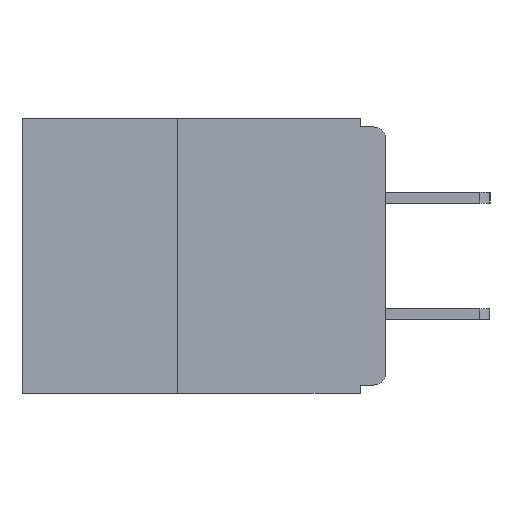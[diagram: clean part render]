
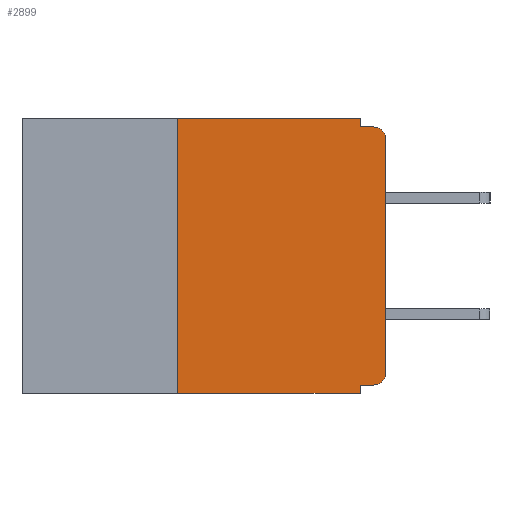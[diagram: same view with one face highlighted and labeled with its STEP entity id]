
A CAD part, left-side view. The second image highlights one B-rep face of the part: STEP entity #2899.
In plain terms, the highlighted planar face has unit normal (-1, 0, 0).
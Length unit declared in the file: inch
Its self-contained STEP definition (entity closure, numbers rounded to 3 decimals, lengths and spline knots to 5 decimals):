
#311 = VECTOR ( 'NONE', #7540, 39.37008 ) ;
#428 = CARTESIAN_POINT ( 'NONE',  ( 0., 0.25, 0. ) ) ;
#472 = VECTOR ( 'NONE', #2282, 39.37008 ) ;
#618 = CARTESIAN_POINT ( 'NONE',  ( 0., 0.015, -0.32 ) ) ;
#641 = VECTOR ( 'NONE', #3483, 39.37008 ) ;
#679 = EDGE_CURVE ( 'NONE', #4457, #3249, #1310, .T. ) ;
#715 = CARTESIAN_POINT ( 'NONE',  ( 0., 0., -0.32 ) ) ;
#743 = ORIENTED_EDGE ( 'NONE', *, *, #795, .T. ) ;
#750 = EDGE_CURVE ( 'NONE', #2171, #4228, #9390, .T. ) ;
#795 = EDGE_CURVE ( 'NONE', #2171, #6616, #3520, .T. ) ;
#797 = LINE ( 'NONE', #11637, #472 ) ;
#818 = EDGE_CURVE ( 'NONE', #1198, #6616, #797, .T. ) ;
#1198 = VERTEX_POINT ( 'NONE', #11765 ) ;
#1310 = LINE ( 'NONE', #1751, #311 ) ;
#1383 = VECTOR ( 'NONE', #2618, 39.37008 ) ;
#1410 = ORIENTED_EDGE ( 'NONE', *, *, #6175, .T. ) ;
#1751 = CARTESIAN_POINT ( 'NONE',  ( 0., 0.031, 0. ) ) ;
#1775 = AXIS2_PLACEMENT_3D ( 'NONE', #5430, #5412, #5399 ) ;
#1803 = VECTOR ( 'NONE', #10834, 39.37008 ) ;
#1867 = LINE ( 'NONE', #715, #9729 ) ;
#2171 = VERTEX_POINT ( 'NONE', #10410 ) ;
#2282 = DIRECTION ( 'NONE',  ( 0., 0., -1. ) ) ;
#2454 = DIRECTION ( 'NONE',  ( -1., 0., 0. ) ) ;
#2488 = CARTESIAN_POINT ( 'NONE',  ( 0., 0.437, 0. ) ) ;
#2618 = DIRECTION ( 'NONE',  ( 0., -1., 0. ) ) ;
#2655 = CARTESIAN_POINT ( 'NONE',  ( 0., 0.031, -0.01 ) ) ;
#2899 = ADVANCED_FACE ( 'NONE', ( #3017 ), #5442, .F. ) ;
#2933 = CARTESIAN_POINT ( 'NONE',  ( 0., 0.25, -0.33 ) ) ;
#3017 = FACE_OUTER_BOUND ( 'NONE', #11963, .T. ) ;
#3060 = VECTOR ( 'NONE', #6805, 39.37008 ) ;
#3136 = VERTEX_POINT ( 'NONE', #3401 ) ;
#3249 = VERTEX_POINT ( 'NONE', #2655 ) ;
#3401 = CARTESIAN_POINT ( 'NONE',  ( 0., 0., -0.305 ) ) ;
#3478 = ORIENTED_EDGE ( 'NONE', *, *, #818, .F. ) ;
#3483 = DIRECTION ( 'NONE',  ( 0., -1., 0. ) ) ;
#3520 = LINE ( 'NONE', #11649, #6071 ) ;
#3541 = CARTESIAN_POINT ( 'NONE',  ( 0., 0.031, -0.33 ) ) ;
#4062 = ORIENTED_EDGE ( 'NONE', *, *, #9400, .T. ) ;
#4228 = VERTEX_POINT ( 'NONE', #428 ) ;
#4290 = CARTESIAN_POINT ( 'NONE',  ( 0., 0.015, -0.305 ) ) ;
#4457 = VERTEX_POINT ( 'NONE', #10857 ) ;
#5075 = AXIS2_PLACEMENT_3D ( 'NONE', #4290, #10738, #5265 ) ;
#5265 = DIRECTION ( 'NONE',  ( 0., 0., -1. ) ) ;
#5294 = ORIENTED_EDGE ( 'NONE', *, *, #10520, .T. ) ;
#5322 = CARTESIAN_POINT ( 'NONE',  ( 0., 0.015, -0.01 ) ) ;
#5399 = DIRECTION ( 'NONE',  ( 0., 0., -1. ) ) ;
#5412 = DIRECTION ( 'NONE',  ( 1., 0., 0. ) ) ;
#5430 = CARTESIAN_POINT ( 'NONE',  ( 0., 0.437, 0. ) ) ;
#5441 = ORIENTED_EDGE ( 'NONE', *, *, #750, .F. ) ;
#5442 = PLANE ( 'NONE',  #1775 ) ;
#5630 = LINE ( 'NONE', #8663, #3060 ) ;
#6071 = VECTOR ( 'NONE', #9850, 39.37008 ) ;
#6175 = EDGE_CURVE ( 'NONE', #3136, #7165, #5630, .T. ) ;
#6616 = VERTEX_POINT ( 'NONE', #3541 ) ;
#6631 = DIRECTION ( 'NONE',  ( 0., 1., 0. ) ) ;
#6805 = DIRECTION ( 'NONE',  ( 0., 0., 1. ) ) ;
#6875 = LINE ( 'NONE', #10138, #1383 ) ;
#7045 = ORIENTED_EDGE ( 'NONE', *, *, #10639, .F. ) ;
#7165 = VERTEX_POINT ( 'NONE', #9878 ) ;
#7174 = ORIENTED_EDGE ( 'NONE', *, *, #679, .F. ) ;
#7386 = EDGE_CURVE ( 'NONE', #3249, #8506, #6875, .T. ) ;
#7540 = DIRECTION ( 'NONE',  ( 0., 0., -1. ) ) ;
#7552 = CIRCLE ( 'NONE', #10906, 0.015 ) ;
#8198 = CARTESIAN_POINT ( 'NONE',  ( 0., 0.015, -0.025 ) ) ;
#8506 = VERTEX_POINT ( 'NONE', #5322 ) ;
#8663 = CARTESIAN_POINT ( 'NONE',  ( 0., 0., 0. ) ) ;
#8858 = EDGE_CURVE ( 'NONE', #11752, #1198, #1867, .T. ) ;
#9009 = LINE ( 'NONE', #2488, #641 ) ;
#9090 = ORIENTED_EDGE ( 'NONE', *, *, #8858, .F. ) ;
#9103 = DIRECTION ( 'NONE',  ( 0., 0., -1. ) ) ;
#9336 = ORIENTED_EDGE ( 'NONE', *, *, #7386, .F. ) ;
#9390 = LINE ( 'NONE', #2933, #1803 ) ;
#9400 = EDGE_CURVE ( 'NONE', #7165, #8506, #7552, .T. ) ;
#9729 = VECTOR ( 'NONE', #6631, 39.37008 ) ;
#9850 = DIRECTION ( 'NONE',  ( 0., -1., 0. ) ) ;
#9878 = CARTESIAN_POINT ( 'NONE',  ( 0., 0., -0.025 ) ) ;
#10138 = CARTESIAN_POINT ( 'NONE',  ( 0., 0., -0.01 ) ) ;
#10410 = CARTESIAN_POINT ( 'NONE',  ( 0., 0.25, -0.33 ) ) ;
#10520 = EDGE_CURVE ( 'NONE', #11752, #3136, #11841, .T. ) ;
#10639 = EDGE_CURVE ( 'NONE', #4228, #4457, #9009, .T. ) ;
#10738 = DIRECTION ( 'NONE',  ( -1., 0., 0. ) ) ;
#10834 = DIRECTION ( 'NONE',  ( 0., 0., 1. ) ) ;
#10857 = CARTESIAN_POINT ( 'NONE',  ( 0., 0.031, 0. ) ) ;
#10906 = AXIS2_PLACEMENT_3D ( 'NONE', #8198, #2454, #9103 ) ;
#11637 = CARTESIAN_POINT ( 'NONE',  ( 0., 0.031, -0.33 ) ) ;
#11649 = CARTESIAN_POINT ( 'NONE',  ( 0., 0.437, -0.33 ) ) ;
#11752 = VERTEX_POINT ( 'NONE', #618 ) ;
#11765 = CARTESIAN_POINT ( 'NONE',  ( 0., 0.031, -0.32 ) ) ;
#11841 = CIRCLE ( 'NONE', #5075, 0.015 ) ;
#11963 = EDGE_LOOP ( 'NONE', ( #1410, #4062, #9336, #7174, #7045, #5441, #743, #3478, #9090, #5294 ) ) ;
